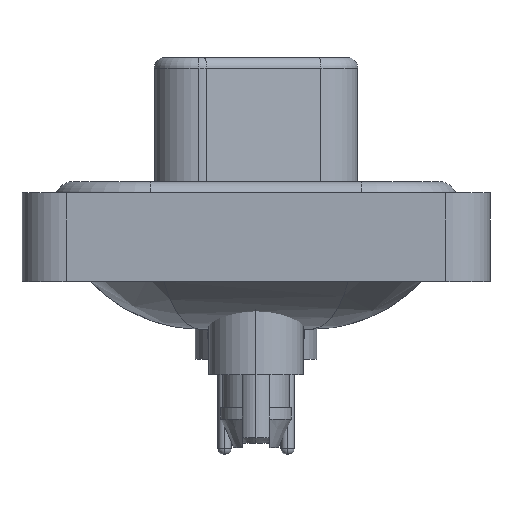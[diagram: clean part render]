
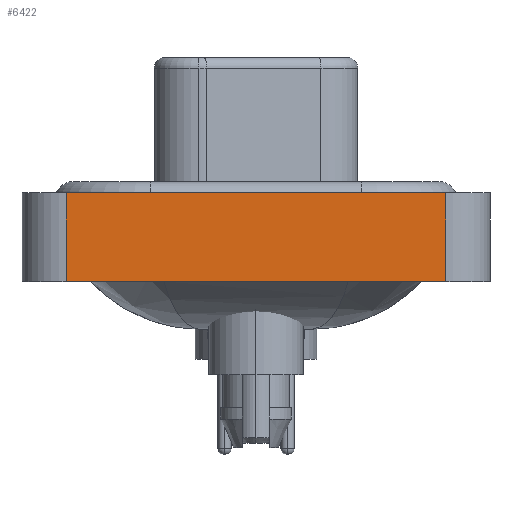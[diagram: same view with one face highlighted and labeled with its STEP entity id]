
A CAD part, left-side view. The second image highlights one B-rep face of the part: STEP entity #6422.
In plain terms, the highlighted planar face has unit normal (-1, 0, 0).
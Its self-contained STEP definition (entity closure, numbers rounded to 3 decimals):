
#117 = PLANE ( 'NONE',  #14264 ) ;
#122 = CARTESIAN_POINT ( 'NONE',  ( -7.25, -8.55, -3.6 ) ) ;
#482 = EDGE_CURVE ( 'NONE', #13357, #8006, #7486, .T. ) ;
#541 = VERTEX_POINT ( 'NONE', #122 ) ;
#666 = VECTOR ( 'NONE', #12640, 1000. ) ;
#1131 = CARTESIAN_POINT ( 'NONE',  ( -7.25, -8.55, -3.6 ) ) ;
#1413 = DIRECTION ( 'NONE',  ( 0., 0., 1. ) ) ;
#1615 = ORIENTED_EDGE ( 'NONE', *, *, #12154, .T. ) ;
#2549 = VECTOR ( 'NONE', #16253, 1000. ) ;
#3531 = EDGE_CURVE ( 'NONE', #8006, #15815, #13078, .T. ) ;
#4413 = DIRECTION ( 'NONE',  ( 0., 0., 1. ) ) ;
#4616 = DIRECTION ( 'NONE',  ( 0., 0., 1. ) ) ;
#5821 = CARTESIAN_POINT ( 'NONE',  ( -7.25, 8.55, -3.6 ) ) ;
#6422 = ADVANCED_FACE ( 'NONE', ( #11431 ), #117, .T. ) ;
#7447 = CARTESIAN_POINT ( 'NONE',  ( -7.25, -8.55, 0.4 ) ) ;
#7486 = LINE ( 'NONE', #5821, #14699 ) ;
#8006 = VERTEX_POINT ( 'NONE', #13212 ) ;
#8086 = ORIENTED_EDGE ( 'NONE', *, *, #12111, .T. ) ;
#8432 = CARTESIAN_POINT ( 'NONE',  ( -7.25, -8.55, -3.6 ) ) ;
#9088 = ORIENTED_EDGE ( 'NONE', *, *, #3531, .F. ) ;
#11138 = LINE ( 'NONE', #16922, #666 ) ;
#11237 = DIRECTION ( 'NONE',  ( -1., 0., 0. ) ) ;
#11431 = FACE_OUTER_BOUND ( 'NONE', #15599, .T. ) ;
#12111 = EDGE_CURVE ( 'NONE', #541, #15815, #15245, .T. ) ;
#12154 = EDGE_CURVE ( 'NONE', #13357, #541, #11138, .T. ) ;
#12220 = CARTESIAN_POINT ( 'NONE',  ( -7.25, -8.55, 0.4 ) ) ;
#12640 = DIRECTION ( 'NONE',  ( 0., -1., 0. ) ) ;
#12981 = ORIENTED_EDGE ( 'NONE', *, *, #482, .F. ) ;
#13078 = LINE ( 'NONE', #7447, #2549 ) ;
#13212 = CARTESIAN_POINT ( 'NONE',  ( -7.25, 8.55, 0.4 ) ) ;
#13357 = VERTEX_POINT ( 'NONE', #17098 ) ;
#14264 = AXIS2_PLACEMENT_3D ( 'NONE', #8432, #11237, #4413 ) ;
#14699 = VECTOR ( 'NONE', #4616, 1000. ) ;
#15245 = LINE ( 'NONE', #1131, #16473 ) ;
#15599 = EDGE_LOOP ( 'NONE', ( #8086, #9088, #12981, #1615 ) ) ;
#15815 = VERTEX_POINT ( 'NONE', #12220 ) ;
#16253 = DIRECTION ( 'NONE',  ( 0., -1., 0. ) ) ;
#16473 = VECTOR ( 'NONE', #1413, 1000. ) ;
#16922 = CARTESIAN_POINT ( 'NONE',  ( -7.25, -8.55, -3.6 ) ) ;
#17098 = CARTESIAN_POINT ( 'NONE',  ( -7.25, 8.55, -3.6 ) ) ;
